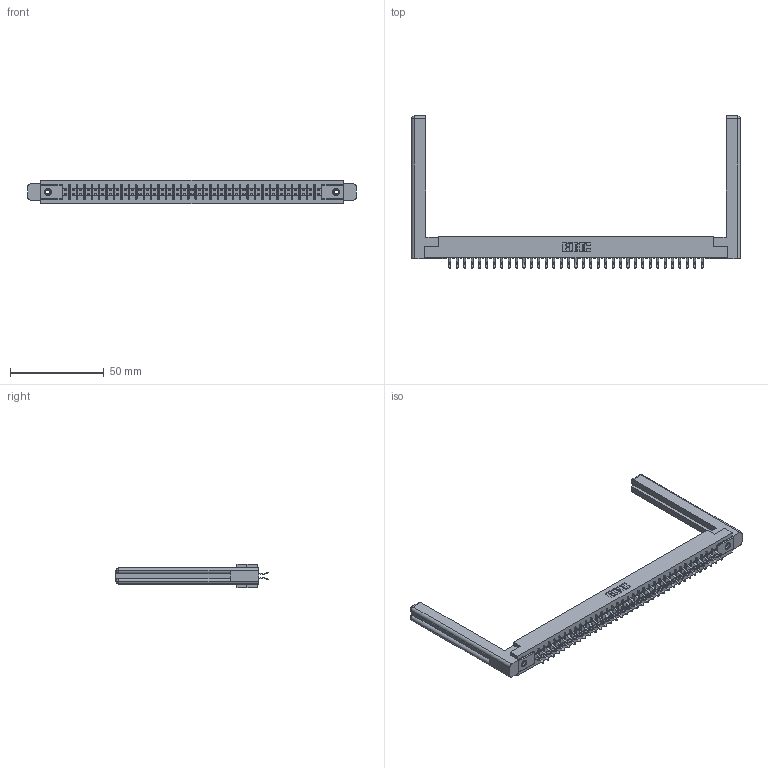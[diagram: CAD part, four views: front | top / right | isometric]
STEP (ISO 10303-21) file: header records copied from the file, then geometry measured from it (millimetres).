
FILE_DESCRIPTION (( 'STEP AP203' ), '1' );
FILE_NAME ('355-070-556-258.STEP', '2019-09-12T17:44:48', ( '' ), ( '' ), 'SwSTEP 2.0', 'SolidWorks 2016', '' );
FILE_SCHEMA (( 'CONFIG_CONTROL_DESIGN' ));
Length unit declared in the file: inch
Products named in the file (5): 345-250-001_345-250-001-102; 305 Part_.156 Dia; 355-070-556-258; 305-290-001_556; 307-220-058
Assembly tree (75 placements, depth 2):
  355-070-556-258
    305 Part_.156 Dia
    305-290-001_556  x70
    345-250-001_345-250-001-102  x2
    307-220-058  x2
Bounding box: 175.31 x 81.28 x 12.7 mm (x, y, z)
Volume: 25388.1 mm3; surface area: 27925.2 mm2
Topology: 75 solids, 75 shells, 4178 faces, 11975 edges, 7782 vertices
Faces by surface type: plane 2322, cylinder 1692, sphere 140, cone 12, torus 12
Entity records: 41603 total; most frequent: CARTESIAN_POINT 6902, ORIENTED_EDGE 6792, DIRECTION 6648, EDGE_CURVE 3396, LINE 2724, VECTOR 2724, VERTEX_POINT 2162, AXIS2_PLACEMENT_3D 1962
